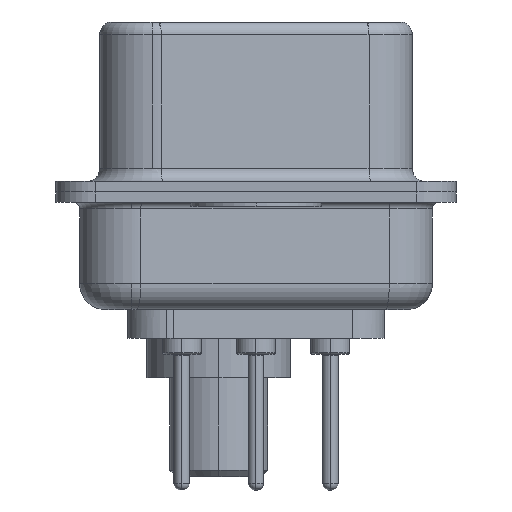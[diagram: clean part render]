
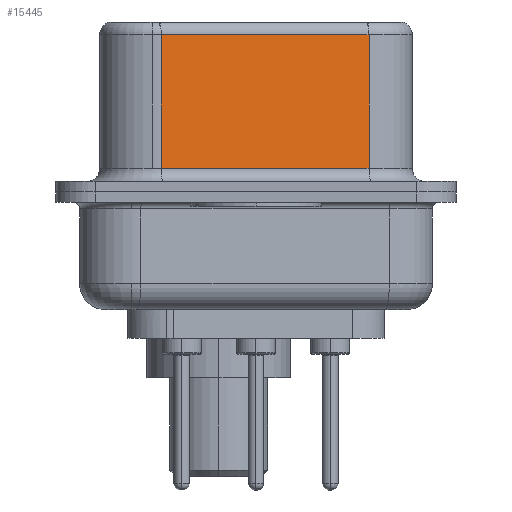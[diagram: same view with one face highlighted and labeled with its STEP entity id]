
A CAD part, left-side view. The second image highlights one B-rep face of the part: STEP entity #15445.
In plain terms, the highlighted planar face has unit normal (-0.985, -0.174, 0).
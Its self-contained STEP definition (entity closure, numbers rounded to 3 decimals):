
#89 = CARTESIAN_POINT ( 'NONE',  ( 5.132, -4.322, 6.52 ) ) ;
#180 = DIRECTION ( 'NONE',  ( -0.174, 0.985, 0. ) ) ;
#657 = CARTESIAN_POINT ( 'NONE',  ( 5.132, -4.322, 6.02 ) ) ;
#2473 = LINE ( 'NONE', #24500, #7603 ) ;
#2498 = LINE ( 'NONE', #6854, #23807 ) ;
#2748 = EDGE_LOOP ( 'NONE', ( #15895, #15696, #24492, #23602 ) ) ;
#3676 = CARTESIAN_POINT ( 'NONE',  ( 5.132, -4.322, 6.52 ) ) ;
#3829 = VERTEX_POINT ( 'NONE', #15736 ) ;
#5869 = CARTESIAN_POINT ( 'NONE',  ( 3.73, 3.628, 0.9 ) ) ;
#6665 = PLANE ( 'NONE',  #23918 ) ;
#6854 = CARTESIAN_POINT ( 'NONE',  ( 5.132, -4.322, 6.02 ) ) ;
#7603 = VECTOR ( 'NONE', #18269, 1000. ) ;
#7662 = VERTEX_POINT ( 'NONE', #22825 ) ;
#8074 = FACE_OUTER_BOUND ( 'NONE', #2748, .T. ) ;
#8774 = DIRECTION ( 'NONE',  ( -0.174, 0.985, 0. ) ) ;
#10062 = EDGE_CURVE ( 'NONE', #26759, #7662, #25681, .T. ) ;
#10107 = EDGE_CURVE ( 'NONE', #20706, #7662, #15753, .T. ) ;
#13746 = VECTOR ( 'NONE', #17500, 1000. ) ;
#15445 = ADVANCED_FACE ( 'NONE', ( #8074 ), #6665, .F. ) ;
#15696 = ORIENTED_EDGE ( 'NONE', *, *, #26050, .T. ) ;
#15736 = CARTESIAN_POINT ( 'NONE',  ( 3.73, 3.628, 6.02 ) ) ;
#15753 = LINE ( 'NONE', #3676, #13746 ) ;
#15895 = ORIENTED_EDGE ( 'NONE', *, *, #10107, .F. ) ;
#17500 = DIRECTION ( 'NONE',  ( 0., 0., -1. ) ) ;
#18269 = DIRECTION ( 'NONE',  ( 0., 0., -1. ) ) ;
#18454 = EDGE_CURVE ( 'NONE', #3829, #26759, #2473, .T. ) ;
#20076 = VECTOR ( 'NONE', #22701, 1000. ) ;
#20706 = VERTEX_POINT ( 'NONE', #657 ) ;
#21443 = DIRECTION ( 'NONE',  ( 0.985, 0.174, 0. ) ) ;
#22701 = DIRECTION ( 'NONE',  ( 0.174, -0.985, 0. ) ) ;
#22825 = CARTESIAN_POINT ( 'NONE',  ( 5.132, -4.322, 0.9 ) ) ;
#23602 = ORIENTED_EDGE ( 'NONE', *, *, #10062, .T. ) ;
#23807 = VECTOR ( 'NONE', #180, 1000. ) ;
#23918 = AXIS2_PLACEMENT_3D ( 'NONE', #89, #21443, #8774 ) ;
#24492 = ORIENTED_EDGE ( 'NONE', *, *, #18454, .T. ) ;
#24500 = CARTESIAN_POINT ( 'NONE',  ( 3.73, 3.628, 6.52 ) ) ;
#25115 = CARTESIAN_POINT ( 'NONE',  ( 5.132, -4.322, 0.9 ) ) ;
#25681 = LINE ( 'NONE', #25115, #20076 ) ;
#26050 = EDGE_CURVE ( 'NONE', #20706, #3829, #2498, .T. ) ;
#26759 = VERTEX_POINT ( 'NONE', #5869 ) ;
